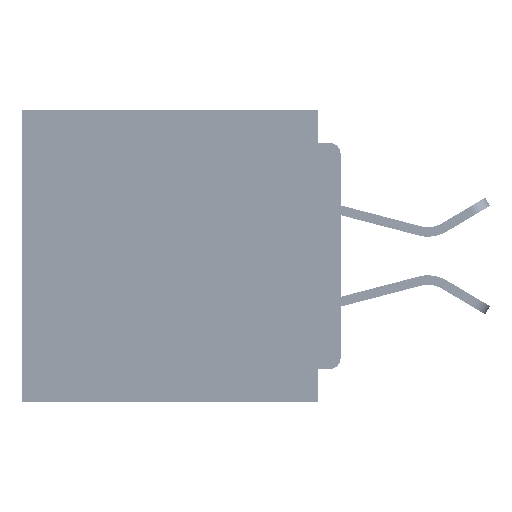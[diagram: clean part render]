
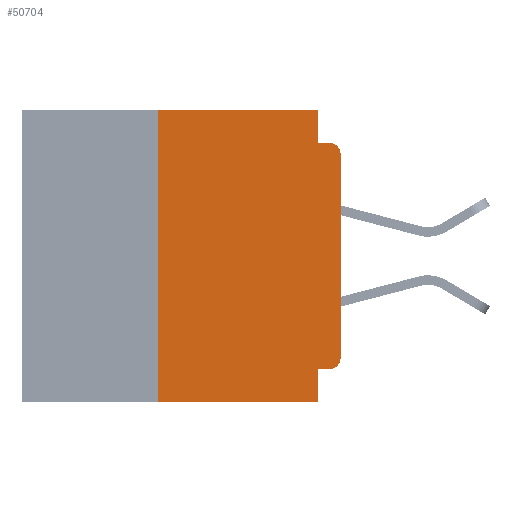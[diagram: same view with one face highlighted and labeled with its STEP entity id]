
A CAD part, left-side view. The second image highlights one B-rep face of the part: STEP entity #50704.
In plain terms, the highlighted planar face has unit normal (-1, 0, 0).
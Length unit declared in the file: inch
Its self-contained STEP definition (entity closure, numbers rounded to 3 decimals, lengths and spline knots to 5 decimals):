
#241 = ORIENTED_EDGE ( 'NONE', *, *, #15531, .F. ) ;
#251 = VERTEX_POINT ( 'NONE', #2501 ) ;
#1877 = PLANE ( 'NONE',  #39080 ) ;
#1916 = CARTESIAN_POINT ( 'NONE',  ( 0., 0.015, -0.355 ) ) ;
#2501 = CARTESIAN_POINT ( 'NONE',  ( 0., 0.25, -0.4 ) ) ;
#2548 = VECTOR ( 'NONE', #29314, 39.37008 ) ;
#2878 = VECTOR ( 'NONE', #48457, 39.37008 ) ;
#3129 = DIRECTION ( 'NONE',  ( 0., -1., 0. ) ) ;
#3697 = AXIS2_PLACEMENT_3D ( 'NONE', #43996, #19138, #48121 ) ;
#4199 = VERTEX_POINT ( 'NONE', #43650 ) ;
#4272 = FACE_OUTER_BOUND ( 'NONE', #37804, .T. ) ;
#4969 = DIRECTION ( 'NONE',  ( 0., 0., -1. ) ) ;
#5087 = LINE ( 'NONE', #35088, #16239 ) ;
#5174 = CARTESIAN_POINT ( 'NONE',  ( 0., 0.031, 0. ) ) ;
#5772 = AXIS2_PLACEMENT_3D ( 'NONE', #10057, #39129, #14248 ) ;
#5808 = VERTEX_POINT ( 'NONE', #37278 ) ;
#5850 = EDGE_CURVE ( 'NONE', #251, #51484, #35819, .T. ) ;
#7330 = CARTESIAN_POINT ( 'NONE',  ( 0., 0.25, 0. ) ) ;
#8491 = VECTOR ( 'NONE', #45884, 39.37008 ) ;
#9199 = CARTESIAN_POINT ( 'NONE',  ( 0., 0.031, -0.4 ) ) ;
#9715 = EDGE_CURVE ( 'NONE', #36457, #46074, #40588, .T. ) ;
#9801 = VERTEX_POINT ( 'NONE', #47351 ) ;
#10057 = CARTESIAN_POINT ( 'NONE',  ( 0., 0.015, -0.06 ) ) ;
#10230 = DIRECTION ( 'NONE',  ( 0., -1., 0. ) ) ;
#10369 = CARTESIAN_POINT ( 'NONE',  ( 0., 0.437, 0. ) ) ;
#11388 = VERTEX_POINT ( 'NONE', #45011 ) ;
#12111 = ORIENTED_EDGE ( 'NONE', *, *, #39105, .T. ) ;
#13775 = ORIENTED_EDGE ( 'NONE', *, *, #9715, .F. ) ;
#14248 = DIRECTION ( 'NONE',  ( 0., 0., -1. ) ) ;
#14554 = DIRECTION ( 'NONE',  ( 0., 0., -1. ) ) ;
#14581 = EDGE_CURVE ( 'NONE', #22317, #11388, #52768, .T. ) ;
#14941 = ORIENTED_EDGE ( 'NONE', *, *, #44709, .T. ) ;
#15531 = EDGE_CURVE ( 'NONE', #4199, #9801, #40446, .T. ) ;
#16239 = VECTOR ( 'NONE', #10230, 39.37008 ) ;
#17036 = VECTOR ( 'NONE', #4969, 39.37008 ) ;
#19117 = ORIENTED_EDGE ( 'NONE', *, *, #36263, .T. ) ;
#19138 = DIRECTION ( 'NONE',  ( -1., 0., 0. ) ) ;
#20158 = VECTOR ( 'NONE', #29536, 39.37008 ) ;
#20573 = EDGE_CURVE ( 'NONE', #46074, #5808, #5087, .T. ) ;
#21185 = CARTESIAN_POINT ( 'NONE',  ( 0., 0., 0. ) ) ;
#22317 = VERTEX_POINT ( 'NONE', #1916 ) ;
#23223 = EDGE_CURVE ( 'NONE', #22317, #4199, #44563, .T. ) ;
#23601 = CARTESIAN_POINT ( 'NONE',  ( 0., 0., -0.355 ) ) ;
#25105 = CARTESIAN_POINT ( 'NONE',  ( 0., 0.25, -0.4 ) ) ;
#27073 = ORIENTED_EDGE ( 'NONE', *, *, #5850, .F. ) ;
#28159 = CARTESIAN_POINT ( 'NONE',  ( 0., 0.437, -0.4 ) ) ;
#28827 = EDGE_CURVE ( 'NONE', #51484, #36457, #41681, .T. ) ;
#29314 = DIRECTION ( 'NONE',  ( 0., 0., 1. ) ) ;
#29340 = ORIENTED_EDGE ( 'NONE', *, *, #28827, .F. ) ;
#29536 = DIRECTION ( 'NONE',  ( 0., 0., 1. ) ) ;
#29551 = VECTOR ( 'NONE', #34301, 39.37008 ) ;
#29597 = VECTOR ( 'NONE', #3129, 39.37008 ) ;
#30548 = ORIENTED_EDGE ( 'NONE', *, *, #23223, .F. ) ;
#32185 = ORIENTED_EDGE ( 'NONE', *, *, #20573, .F. ) ;
#34301 = DIRECTION ( 'NONE',  ( 0., 0., -1. ) ) ;
#35088 = CARTESIAN_POINT ( 'NONE',  ( 0., 0., -0.045 ) ) ;
#35819 = LINE ( 'NONE', #25105, #2548 ) ;
#35888 = ORIENTED_EDGE ( 'NONE', *, *, #14581, .T. ) ;
#35945 = CIRCLE ( 'NONE', #5772, 0.015 ) ;
#36263 = EDGE_CURVE ( 'NONE', #251, #9801, #40624, .T. ) ;
#36457 = VERTEX_POINT ( 'NONE', #37728 ) ;
#37278 = CARTESIAN_POINT ( 'NONE',  ( 0., 0.015, -0.045 ) ) ;
#37450 = VERTEX_POINT ( 'NONE', #43113 ) ;
#37728 = CARTESIAN_POINT ( 'NONE',  ( 0., 0.031, 0. ) ) ;
#37804 = EDGE_LOOP ( 'NONE', ( #12111, #14941, #32185, #13775, #29340, #27073, #19117, #241, #30548, #35888 ) ) ;
#39080 = AXIS2_PLACEMENT_3D ( 'NONE', #10369, #39440, #14554 ) ;
#39105 = EDGE_CURVE ( 'NONE', #11388, #37450, #53154, .T. ) ;
#39129 = DIRECTION ( 'NONE',  ( -1., 0., 0. ) ) ;
#39440 = DIRECTION ( 'NONE',  ( 1., 0., 0. ) ) ;
#40446 = LINE ( 'NONE', #9199, #17036 ) ;
#40588 = LINE ( 'NONE', #5174, #29551 ) ;
#40624 = LINE ( 'NONE', #28159, #29597 ) ;
#41681 = LINE ( 'NONE', #41755, #8491 ) ;
#41755 = CARTESIAN_POINT ( 'NONE',  ( 0., 0.437, 0. ) ) ;
#43113 = CARTESIAN_POINT ( 'NONE',  ( 0., 0., -0.06 ) ) ;
#43650 = CARTESIAN_POINT ( 'NONE',  ( 0., 0.031, -0.355 ) ) ;
#43996 = CARTESIAN_POINT ( 'NONE',  ( 0., 0.015, -0.34 ) ) ;
#44563 = LINE ( 'NONE', #23601, #2878 ) ;
#44709 = EDGE_CURVE ( 'NONE', #37450, #5808, #35945, .T. ) ;
#45011 = CARTESIAN_POINT ( 'NONE',  ( 0., 0., -0.34 ) ) ;
#45884 = DIRECTION ( 'NONE',  ( 0., -1., 0. ) ) ;
#46074 = VERTEX_POINT ( 'NONE', #51253 ) ;
#47351 = CARTESIAN_POINT ( 'NONE',  ( 0., 0.031, -0.4 ) ) ;
#48121 = DIRECTION ( 'NONE',  ( 0., 0., -1. ) ) ;
#48457 = DIRECTION ( 'NONE',  ( 0., 1., 0. ) ) ;
#50704 = ADVANCED_FACE ( 'NONE', ( #4272 ), #1877, .F. ) ;
#51253 = CARTESIAN_POINT ( 'NONE',  ( 0., 0.031, -0.045 ) ) ;
#51484 = VERTEX_POINT ( 'NONE', #7330 ) ;
#52768 = CIRCLE ( 'NONE', #3697, 0.015 ) ;
#53154 = LINE ( 'NONE', #21185, #20158 ) ;
